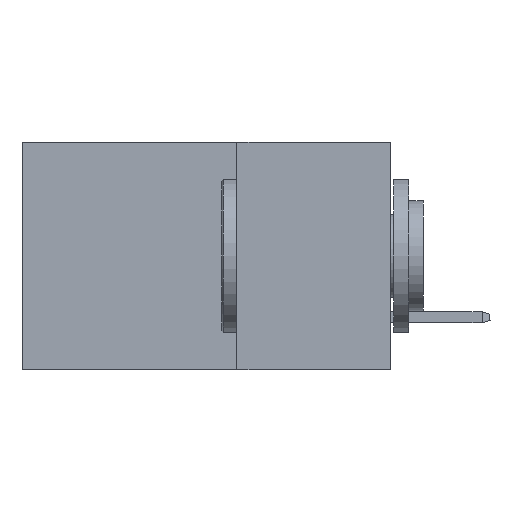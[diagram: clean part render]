
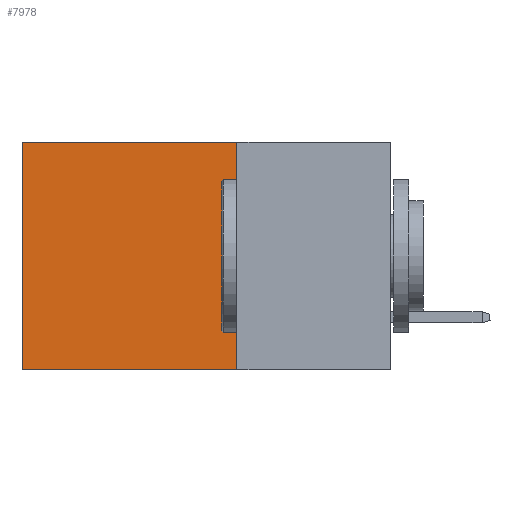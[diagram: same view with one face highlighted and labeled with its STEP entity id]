
A CAD part, left-side view. The second image highlights one B-rep face of the part: STEP entity #7978.
In plain terms, the highlighted planar face has unit normal (-1, 0, 0).
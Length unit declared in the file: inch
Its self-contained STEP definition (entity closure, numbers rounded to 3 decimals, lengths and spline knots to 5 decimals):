
#286 = CARTESIAN_POINT ( 'NONE',  ( 0.2875, 0.6, 0. ) ) ;
#301 = LINE ( 'NONE', #1944, #9448 ) ;
#792 = PLANE ( 'NONE',  #2345 ) ;
#877 = EDGE_CURVE ( 'NONE', #1251, #3758, #6255, .T. ) ;
#1062 = LINE ( 'NONE', #8414, #9814 ) ;
#1251 = VERTEX_POINT ( 'NONE', #1794 ) ;
#1433 = DIRECTION ( 'NONE',  ( 0., 1., 0. ) ) ;
#1565 = CARTESIAN_POINT ( 'NONE',  ( 0.2875, 0.6, -0.37 ) ) ;
#1794 = CARTESIAN_POINT ( 'NONE',  ( 0.2875, 0.25, 0. ) ) ;
#1944 = CARTESIAN_POINT ( 'NONE',  ( 0.2875, 0.25, 0. ) ) ;
#2345 = AXIS2_PLACEMENT_3D ( 'NONE', #8906, #8882, #9673 ) ;
#2618 = CARTESIAN_POINT ( 'NONE',  ( 0.2875, 0.6, 0. ) ) ;
#2802 = EDGE_CURVE ( 'NONE', #3758, #7470, #8531, .T. ) ;
#3758 = VERTEX_POINT ( 'NONE', #286 ) ;
#4026 = EDGE_CURVE ( 'NONE', #6391, #7470, #1062, .T. ) ;
#5086 = EDGE_CURVE ( 'NONE', #1251, #6391, #301, .T. ) ;
#5249 = DIRECTION ( 'NONE',  ( 0., 1., 0. ) ) ;
#5573 = ORIENTED_EDGE ( 'NONE', *, *, #5086, .F. ) ;
#5671 = ORIENTED_EDGE ( 'NONE', *, *, #2802, .T. ) ;
#5745 = VECTOR ( 'NONE', #5249, 39.37008 ) ;
#5795 = DIRECTION ( 'NONE',  ( 0., 0., -1. ) ) ;
#6255 = LINE ( 'NONE', #8278, #5745 ) ;
#6328 = ORIENTED_EDGE ( 'NONE', *, *, #4026, .F. ) ;
#6391 = VERTEX_POINT ( 'NONE', #6716 ) ;
#6716 = CARTESIAN_POINT ( 'NONE',  ( 0.2875, 0.25, -0.37 ) ) ;
#7319 = VECTOR ( 'NONE', #8808, 39.37008 ) ;
#7470 = VERTEX_POINT ( 'NONE', #1565 ) ;
#7978 = ADVANCED_FACE ( 'NONE', ( #9457 ), #792, .F. ) ;
#8278 = CARTESIAN_POINT ( 'NONE',  ( 0.2875, 0.25, 0. ) ) ;
#8325 = EDGE_LOOP ( 'NONE', ( #5671, #6328, #5573, #8886 ) ) ;
#8414 = CARTESIAN_POINT ( 'NONE',  ( 0.2875, 0.25, -0.37 ) ) ;
#8531 = LINE ( 'NONE', #2618, #7319 ) ;
#8808 = DIRECTION ( 'NONE',  ( 0., 0., -1. ) ) ;
#8882 = DIRECTION ( 'NONE',  ( 1., 0., 0. ) ) ;
#8886 = ORIENTED_EDGE ( 'NONE', *, *, #877, .T. ) ;
#8906 = CARTESIAN_POINT ( 'NONE',  ( 0.2875, 0.25, 0. ) ) ;
#9448 = VECTOR ( 'NONE', #5795, 39.37008 ) ;
#9457 = FACE_OUTER_BOUND ( 'NONE', #8325, .T. ) ;
#9673 = DIRECTION ( 'NONE',  ( 0., 0., -1. ) ) ;
#9814 = VECTOR ( 'NONE', #1433, 39.37008 ) ;
